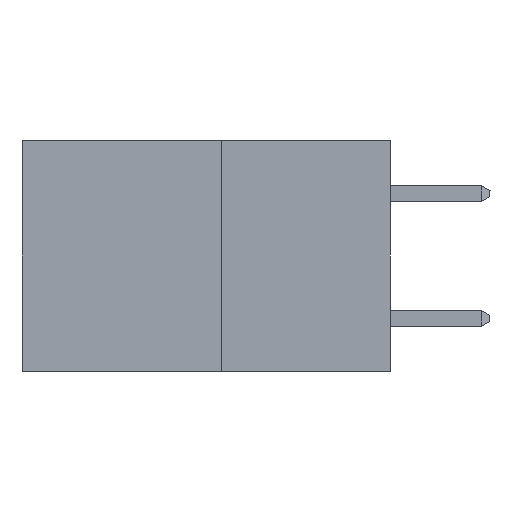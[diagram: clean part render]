
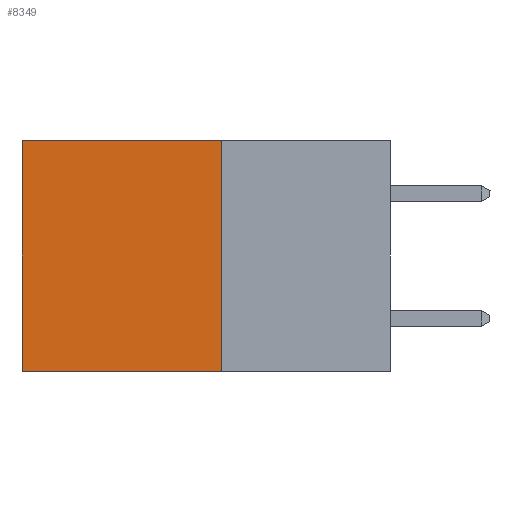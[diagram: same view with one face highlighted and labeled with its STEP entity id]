
A CAD part, left-side view. The second image highlights one B-rep face of the part: STEP entity #8349.
In plain terms, the highlighted planar face has unit normal (-1, 0, 0).
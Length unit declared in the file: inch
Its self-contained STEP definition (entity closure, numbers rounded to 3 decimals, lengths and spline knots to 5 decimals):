
#319 = LINE ( 'NONE', #1800, #6748 ) ;
#366 = CARTESIAN_POINT ( 'NONE',  ( 0.277, 0.27, -0.37 ) ) ;
#523 = CARTESIAN_POINT ( 'NONE',  ( 0.277, 0.27, 0. ) ) ;
#1543 = EDGE_CURVE ( 'NONE', #7794, #8610, #3637, .T. ) ;
#1603 = ORIENTED_EDGE ( 'NONE', *, *, #1543, .T. ) ;
#1800 = CARTESIAN_POINT ( 'NONE',  ( 0.277, 0.27, 0. ) ) ;
#1832 = ORIENTED_EDGE ( 'NONE', *, *, #2121, .T. ) ;
#1988 = FACE_OUTER_BOUND ( 'NONE', #9785, .T. ) ;
#2109 = CARTESIAN_POINT ( 'NONE',  ( 0.277, 0.27, -0.37 ) ) ;
#2121 = EDGE_CURVE ( 'NONE', #2334, #7794, #319, .T. ) ;
#2182 = VERTEX_POINT ( 'NONE', #2662 ) ;
#2334 = VERTEX_POINT ( 'NONE', #523 ) ;
#2662 = CARTESIAN_POINT ( 'NONE',  ( 0.277, 0.27, -0.37 ) ) ;
#2721 = DIRECTION ( 'NONE',  ( 0., 1., 0. ) ) ;
#2959 = EDGE_CURVE ( 'NONE', #2182, #8610, #7233, .T. ) ;
#3421 = CARTESIAN_POINT ( 'NONE',  ( 0.277, 0.59, -0.37 ) ) ;
#3637 = LINE ( 'NONE', #3421, #7765 ) ;
#3687 = EDGE_CURVE ( 'NONE', #2334, #2182, #9345, .T. ) ;
#3734 = PLANE ( 'NONE',  #4111 ) ;
#4111 = AXIS2_PLACEMENT_3D ( 'NONE', #8450, #10006, #5314 ) ;
#4382 = CARTESIAN_POINT ( 'NONE',  ( 0.277, 0.59, 0. ) ) ;
#5091 = DIRECTION ( 'NONE',  ( 0., 0., -1. ) ) ;
#5314 = DIRECTION ( 'NONE',  ( 0., 0., -1. ) ) ;
#5745 = CARTESIAN_POINT ( 'NONE',  ( 0.277, 0.59, -0.37 ) ) ;
#6748 = VECTOR ( 'NONE', #7241, 39.37008 ) ;
#6977 = VECTOR ( 'NONE', #2721, 39.37008 ) ;
#7233 = LINE ( 'NONE', #366, #6977 ) ;
#7241 = DIRECTION ( 'NONE',  ( 0., 1., 0. ) ) ;
#7765 = VECTOR ( 'NONE', #5091, 39.37008 ) ;
#7794 = VERTEX_POINT ( 'NONE', #4382 ) ;
#7812 = ORIENTED_EDGE ( 'NONE', *, *, #2959, .F. ) ;
#8349 = ADVANCED_FACE ( 'NONE', ( #1988 ), #3734, .F. ) ;
#8450 = CARTESIAN_POINT ( 'NONE',  ( 0.277, 0.27, -0.37 ) ) ;
#8610 = VERTEX_POINT ( 'NONE', #5745 ) ;
#9105 = VECTOR ( 'NONE', #9165, 39.37008 ) ;
#9165 = DIRECTION ( 'NONE',  ( 0., 0., -1. ) ) ;
#9345 = LINE ( 'NONE', #2109, #9105 ) ;
#9785 = EDGE_LOOP ( 'NONE', ( #1603, #7812, #9908, #1832 ) ) ;
#9908 = ORIENTED_EDGE ( 'NONE', *, *, #3687, .F. ) ;
#10006 = DIRECTION ( 'NONE',  ( 1., 0., 0. ) ) ;
